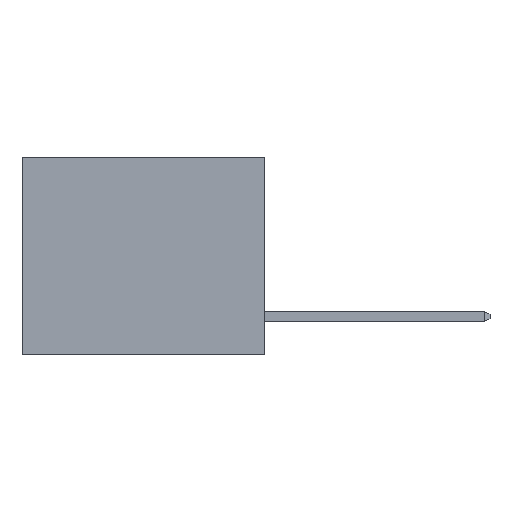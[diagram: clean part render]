
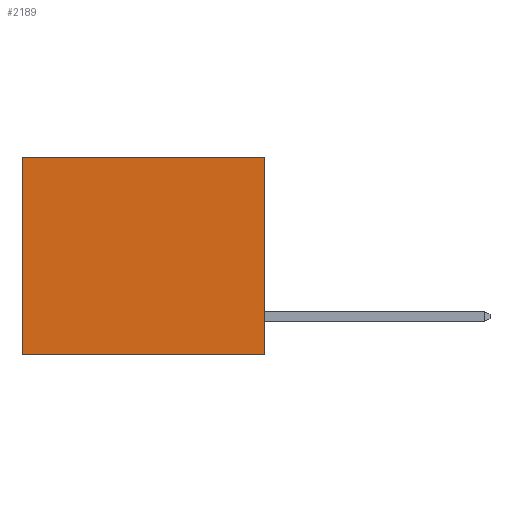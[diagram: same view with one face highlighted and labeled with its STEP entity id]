
A CAD part, left-side view. The second image highlights one B-rep face of the part: STEP entity #2189.
In plain terms, the highlighted planar face has unit normal (-1, 0, 0).
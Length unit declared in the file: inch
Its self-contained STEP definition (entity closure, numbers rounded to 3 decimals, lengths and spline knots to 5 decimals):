
#554 = ORIENTED_EDGE ( 'NONE', *, *, #6167, .T. ) ;
#1247 = EDGE_CURVE ( 'NONE', #7713, #10749, #9448, .T. ) ;
#1538 = PLANE ( 'NONE',  #11035 ) ;
#1696 = CARTESIAN_POINT ( 'NONE',  ( 0.3165, 0.6, -0.49 ) ) ;
#1822 = LINE ( 'NONE', #6101, #8973 ) ;
#2189 = ADVANCED_FACE ( 'NONE', ( #4618 ), #1538, .F. ) ;
#2334 = VECTOR ( 'NONE', #4016, 39.37008 ) ;
#2389 = CARTESIAN_POINT ( 'NONE',  ( 0.3165, 0., -0.49 ) ) ;
#2857 = CARTESIAN_POINT ( 'NONE',  ( 0.3165, 0., -0.49 ) ) ;
#3566 = EDGE_CURVE ( 'NONE', #9403, #7713, #10588, .T. ) ;
#4016 = DIRECTION ( 'NONE',  ( 0., 0., -1. ) ) ;
#4618 = FACE_OUTER_BOUND ( 'NONE', #5972, .T. ) ;
#4852 = DIRECTION ( 'NONE',  ( 1., 0., 0. ) ) ;
#5197 = DIRECTION ( 'NONE',  ( 0., 1., 0. ) ) ;
#5621 = CARTESIAN_POINT ( 'NONE',  ( 0.3165, 0., 0. ) ) ;
#5972 = EDGE_LOOP ( 'NONE', ( #8435, #9925, #9703, #554 ) ) ;
#6101 = CARTESIAN_POINT ( 'NONE',  ( 0.3165, 0., 0. ) ) ;
#6167 = EDGE_CURVE ( 'NONE', #9403, #11168, #1822, .T. ) ;
#6311 = DIRECTION ( 'NONE',  ( 0., 1., 0. ) ) ;
#6583 = CARTESIAN_POINT ( 'NONE',  ( 0.3165, 0., -0.49 ) ) ;
#6796 = DIRECTION ( 'NONE',  ( 0., 0., -1. ) ) ;
#7153 = LINE ( 'NONE', #1696, #2334 ) ;
#7423 = DIRECTION ( 'NONE',  ( 0., 0., -1. ) ) ;
#7583 = CARTESIAN_POINT ( 'NONE',  ( 0.3165, 0.6, -0.49 ) ) ;
#7713 = VERTEX_POINT ( 'NONE', #6583 ) ;
#8435 = ORIENTED_EDGE ( 'NONE', *, *, #10374, .T. ) ;
#8973 = VECTOR ( 'NONE', #5197, 39.37008 ) ;
#9403 = VERTEX_POINT ( 'NONE', #5621 ) ;
#9448 = LINE ( 'NONE', #2389, #10508 ) ;
#9703 = ORIENTED_EDGE ( 'NONE', *, *, #3566, .F. ) ;
#9925 = ORIENTED_EDGE ( 'NONE', *, *, #1247, .F. ) ;
#10342 = CARTESIAN_POINT ( 'NONE',  ( 0.3165, 0., -0.49 ) ) ;
#10374 = EDGE_CURVE ( 'NONE', #11168, #10749, #7153, .T. ) ;
#10508 = VECTOR ( 'NONE', #6311, 39.37008 ) ;
#10588 = LINE ( 'NONE', #10342, #11230 ) ;
#10749 = VERTEX_POINT ( 'NONE', #7583 ) ;
#11035 = AXIS2_PLACEMENT_3D ( 'NONE', #2857, #4852, #6796 ) ;
#11168 = VERTEX_POINT ( 'NONE', #12895 ) ;
#11230 = VECTOR ( 'NONE', #7423, 39.37008 ) ;
#12895 = CARTESIAN_POINT ( 'NONE',  ( 0.3165, 0.6, 0. ) ) ;
